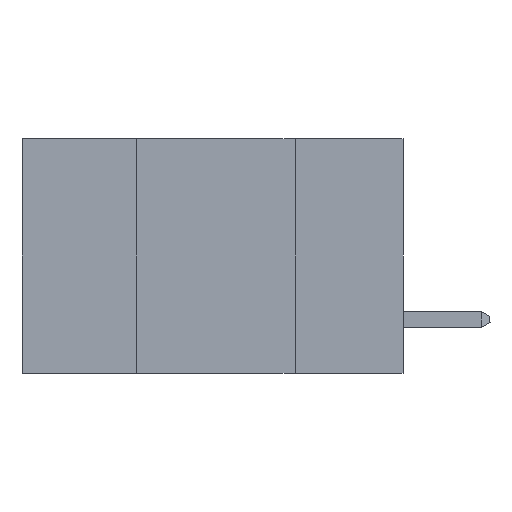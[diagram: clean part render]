
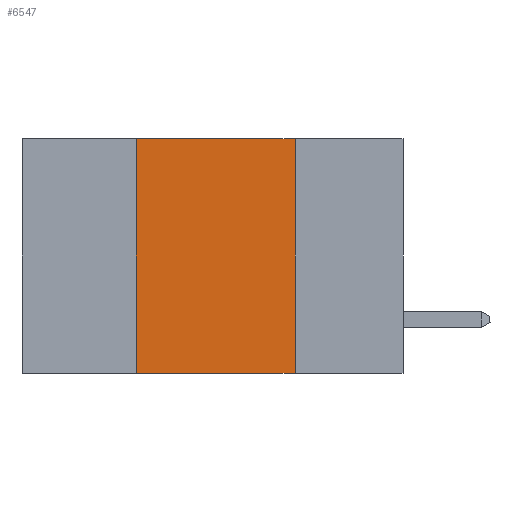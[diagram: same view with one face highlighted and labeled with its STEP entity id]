
A CAD part, left-side view. The second image highlights one B-rep face of the part: STEP entity #6547.
In plain terms, the highlighted planar face has unit normal (-1, 0, 0).
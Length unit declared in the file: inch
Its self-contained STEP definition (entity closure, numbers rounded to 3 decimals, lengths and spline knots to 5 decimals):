
#1816 = DIRECTION ( 'NONE',  ( 0., 0., -1. ) ) ;
#1879 = VECTOR ( 'NONE', #6756, 39.37008 ) ;
#1960 = VECTOR ( 'NONE', #4816, 39.37008 ) ;
#2113 = CARTESIAN_POINT ( 'NONE',  ( 0., 0.17, 0. ) ) ;
#2436 = VERTEX_POINT ( 'NONE', #9495 ) ;
#2657 = DIRECTION ( 'NONE',  ( 1., 0., 0. ) ) ;
#3193 = ORIENTED_EDGE ( 'NONE', *, *, #8164, .F. ) ;
#3607 = LINE ( 'NONE', #11475, #12034 ) ;
#3704 = VERTEX_POINT ( 'NONE', #9442 ) ;
#3989 = DIRECTION ( 'NONE',  ( 0., 0., -1. ) ) ;
#4210 = AXIS2_PLACEMENT_3D ( 'NONE', #11526, #2657, #3989 ) ;
#4292 = EDGE_CURVE ( 'NONE', #3704, #2436, #8333, .T. ) ;
#4816 = DIRECTION ( 'NONE',  ( 0., -1., 0. ) ) ;
#6134 = FACE_OUTER_BOUND ( 'NONE', #16209, .T. ) ;
#6421 = DIRECTION ( 'NONE',  ( 0., -1., 0. ) ) ;
#6525 = EDGE_CURVE ( 'NONE', #3704, #11584, #3607, .T. ) ;
#6547 = ADVANCED_FACE ( 'NONE', ( #6134 ), #9041, .F. ) ;
#6756 = DIRECTION ( 'NONE',  ( 0., 0., 1. ) ) ;
#7777 = EDGE_CURVE ( 'NONE', #11984, #11584, #15327, .T. ) ;
#7845 = LINE ( 'NONE', #13622, #1960 ) ;
#7892 = ORIENTED_EDGE ( 'NONE', *, *, #4292, .F. ) ;
#8164 = EDGE_CURVE ( 'NONE', #2436, #11984, #7845, .T. ) ;
#8333 = LINE ( 'NONE', #14284, #1879 ) ;
#9041 = PLANE ( 'NONE',  #4210 ) ;
#9442 = CARTESIAN_POINT ( 'NONE',  ( 0., 0.42, -0.37 ) ) ;
#9495 = CARTESIAN_POINT ( 'NONE',  ( 0., 0.42, 0. ) ) ;
#11448 = ORIENTED_EDGE ( 'NONE', *, *, #6525, .T. ) ;
#11475 = CARTESIAN_POINT ( 'NONE',  ( 0., 0.6, -0.37 ) ) ;
#11526 = CARTESIAN_POINT ( 'NONE',  ( 0., 0.6, 0. ) ) ;
#11584 = VERTEX_POINT ( 'NONE', #13202 ) ;
#11984 = VERTEX_POINT ( 'NONE', #2113 ) ;
#11995 = VECTOR ( 'NONE', #1816, 39.37008 ) ;
#12034 = VECTOR ( 'NONE', #6421, 39.37008 ) ;
#12400 = ORIENTED_EDGE ( 'NONE', *, *, #7777, .F. ) ;
#13202 = CARTESIAN_POINT ( 'NONE',  ( 0., 0.17, -0.37 ) ) ;
#13622 = CARTESIAN_POINT ( 'NONE',  ( 0., 0.6, 0. ) ) ;
#14143 = CARTESIAN_POINT ( 'NONE',  ( 0., 0.17, 0. ) ) ;
#14284 = CARTESIAN_POINT ( 'NONE',  ( 0., 0.42, 0. ) ) ;
#15327 = LINE ( 'NONE', #14143, #11995 ) ;
#16209 = EDGE_LOOP ( 'NONE', ( #12400, #3193, #7892, #11448 ) ) ;
